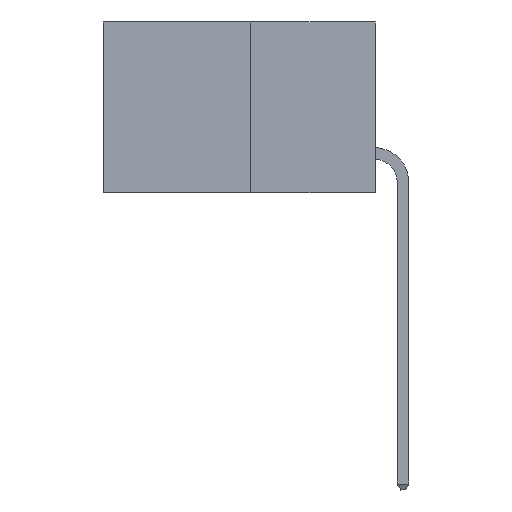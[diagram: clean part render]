
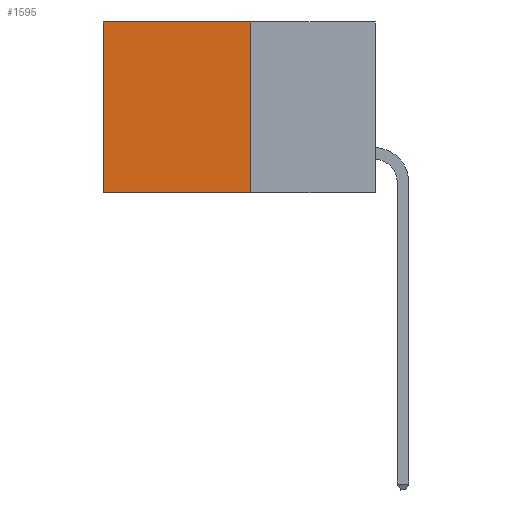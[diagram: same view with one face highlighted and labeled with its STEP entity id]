
A CAD part, left-side view. The second image highlights one B-rep face of the part: STEP entity #1595.
In plain terms, the highlighted planar face has unit normal (-1, 0, 0).
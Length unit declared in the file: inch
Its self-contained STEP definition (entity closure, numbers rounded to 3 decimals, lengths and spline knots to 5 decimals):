
#64 = LINE ( 'NONE', #9662, #3022 ) ;
#305 = LINE ( 'NONE', #4105, #5666 ) ;
#386 = CARTESIAN_POINT ( 'NONE',  ( 0.277, 0.27, 0. ) ) ;
#469 = CARTESIAN_POINT ( 'NONE',  ( 0.277, 0.59, -0.37 ) ) ;
#590 = VERTEX_POINT ( 'NONE', #7518 ) ;
#914 = CARTESIAN_POINT ( 'NONE',  ( 0.277, 0.59, -0.37 ) ) ;
#925 = VECTOR ( 'NONE', #9183, 39.37008 ) ;
#1595 = ADVANCED_FACE ( 'NONE', ( #7886 ), #10059, .F. ) ;
#2280 = DIRECTION ( 'NONE',  ( 0., 0., -1. ) ) ;
#2292 = DIRECTION ( 'NONE',  ( 1., 0., 0. ) ) ;
#2335 = CARTESIAN_POINT ( 'NONE',  ( 0.277, 0.27, -0.37 ) ) ;
#2754 = DIRECTION ( 'NONE',  ( 0., 1., 0. ) ) ;
#3022 = VECTOR ( 'NONE', #9646, 39.37008 ) ;
#3025 = EDGE_CURVE ( 'NONE', #4645, #590, #64, .T. ) ;
#3533 = EDGE_LOOP ( 'NONE', ( #9192, #7193, #7694, #3652 ) ) ;
#3652 = ORIENTED_EDGE ( 'NONE', *, *, #5225, .T. ) ;
#4105 = CARTESIAN_POINT ( 'NONE',  ( 0.277, 0.27, 0. ) ) ;
#4163 = CARTESIAN_POINT ( 'NONE',  ( 0.277, 0.59, 0. ) ) ;
#4645 = VERTEX_POINT ( 'NONE', #386 ) ;
#5225 = EDGE_CURVE ( 'NONE', #4645, #8056, #305, .T. ) ;
#5666 = VECTOR ( 'NONE', #2754, 39.37008 ) ;
#5807 = AXIS2_PLACEMENT_3D ( 'NONE', #2335, #2292, #2280 ) ;
#6196 = LINE ( 'NONE', #8237, #925 ) ;
#7193 = ORIENTED_EDGE ( 'NONE', *, *, #9142, .F. ) ;
#7426 = VECTOR ( 'NONE', #8679, 39.37008 ) ;
#7518 = CARTESIAN_POINT ( 'NONE',  ( 0.277, 0.27, -0.37 ) ) ;
#7694 = ORIENTED_EDGE ( 'NONE', *, *, #3025, .F. ) ;
#7713 = EDGE_CURVE ( 'NONE', #8056, #8077, #12027, .T. ) ;
#7886 = FACE_OUTER_BOUND ( 'NONE', #3533, .T. ) ;
#8056 = VERTEX_POINT ( 'NONE', #4163 ) ;
#8077 = VERTEX_POINT ( 'NONE', #914 ) ;
#8237 = CARTESIAN_POINT ( 'NONE',  ( 0.277, 0.27, -0.37 ) ) ;
#8679 = DIRECTION ( 'NONE',  ( 0., 0., -1. ) ) ;
#9142 = EDGE_CURVE ( 'NONE', #590, #8077, #6196, .T. ) ;
#9183 = DIRECTION ( 'NONE',  ( 0., 1., 0. ) ) ;
#9192 = ORIENTED_EDGE ( 'NONE', *, *, #7713, .T. ) ;
#9646 = DIRECTION ( 'NONE',  ( 0., 0., -1. ) ) ;
#9662 = CARTESIAN_POINT ( 'NONE',  ( 0.277, 0.27, -0.37 ) ) ;
#10059 = PLANE ( 'NONE',  #5807 ) ;
#12027 = LINE ( 'NONE', #469, #7426 ) ;
